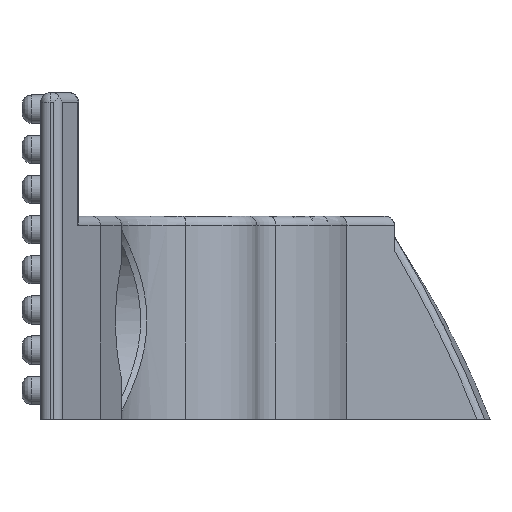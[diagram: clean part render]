
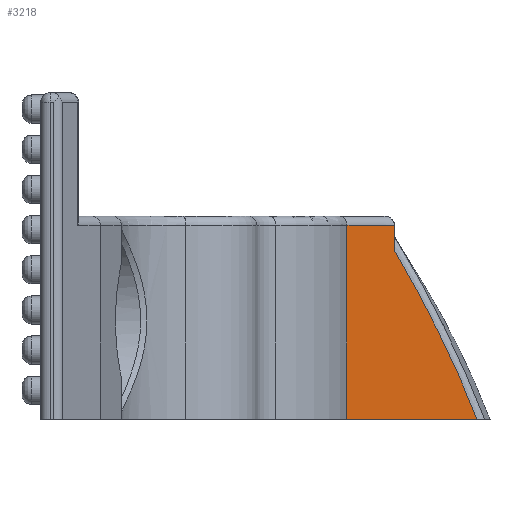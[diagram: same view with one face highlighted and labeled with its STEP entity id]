
A CAD part, left-side view. The second image highlights one B-rep face of the part: STEP entity #3218.
In plain terms, the highlighted planar face has unit normal (-1, 0, 0).
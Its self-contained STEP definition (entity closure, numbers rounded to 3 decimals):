
#130=PLANE('',#3462);
#209=LINE('',#5249,#343);
#210=LINE('',#5251,#344);
#211=LINE('',#5253,#345);
#212=LINE('',#5254,#346);
#343=VECTOR('',#3982,10.);
#344=VECTOR('',#3983,10.);
#345=VECTOR('',#3984,10.);
#346=VECTOR('',#3985,10.);
#789=FACE_OUTER_BOUND('',#1013,.T.);
#1013=EDGE_LOOP('',(#2164,#2165,#2166,#2167,#2168));
#1313=ELLIPSE('',#3461,57.275,51.169);
#1339=VERTEX_POINT('',#5176);
#1340=VERTEX_POINT('',#5208);
#1341=VERTEX_POINT('',#5248);
#1342=VERTEX_POINT('',#5250);
#1343=VERTEX_POINT('',#5252);
#1662=EDGE_CURVE('',#1340,#1339,#1313,.T.);
#1663=EDGE_CURVE('',#1340,#1341,#209,.T.);
#1664=EDGE_CURVE('',#1342,#1341,#210,.T.);
#1665=EDGE_CURVE('',#1342,#1343,#211,.T.);
#1666=EDGE_CURVE('',#1339,#1343,#212,.T.);
#2164=ORIENTED_EDGE('',*,*,#1662,.F.);
#2165=ORIENTED_EDGE('',*,*,#1663,.T.);
#2166=ORIENTED_EDGE('',*,*,#1664,.F.);
#2167=ORIENTED_EDGE('',*,*,#1665,.T.);
#2168=ORIENTED_EDGE('',*,*,#1666,.F.);
#3218=ADVANCED_FACE('',(#789),#130,.T.);
#3461=AXIS2_PLACEMENT_3D('',#5246,#3978,#3979);
#3462=AXIS2_PLACEMENT_3D('',#5247,#3980,#3981);
#3978=DIRECTION('center_axis',(1.,0.,0.));
#3979=DIRECTION('ref_axis',(0.,-0.519,-0.855));
#3980=DIRECTION('center_axis',(-1.,0.,0.));
#3981=DIRECTION('ref_axis',(0.,0.,1.));
#3982=DIRECTION('',(0.,0.,1.));
#3983=DIRECTION('',(0.,-1.,0.));
#3984=DIRECTION('',(0.,0.,-1.));
#3985=DIRECTION('',(0.,1.,0.));
#5176=CARTESIAN_POINT('',(46.9,20.308,57.8));
#5208=CARTESIAN_POINT('',(46.9,24.7,66.788));
#5246=CARTESIAN_POINT('Origin',(46.9,68.859,40.936));
#5247=CARTESIAN_POINT('Origin',(46.9,27.491,57.5));
#5248=CARTESIAN_POINT('',(46.9,24.7,68.1));
#5249=CARTESIAN_POINT('',(46.9,24.7,59.318));
#5250=CARTESIAN_POINT('',(46.9,27.221,68.1));
#5251=CARTESIAN_POINT('',(46.9,31.057,68.1));
#5252=CARTESIAN_POINT('',(46.9,27.221,57.8));
#5253=CARTESIAN_POINT('',(46.9,27.221,68.6));
#5254=CARTESIAN_POINT('',(46.9,31.057,57.8));
